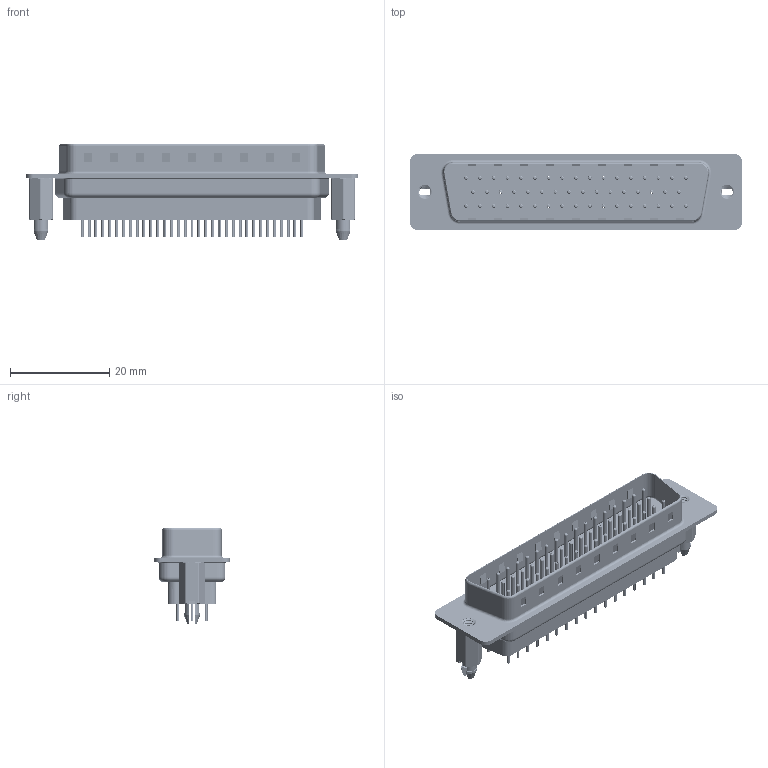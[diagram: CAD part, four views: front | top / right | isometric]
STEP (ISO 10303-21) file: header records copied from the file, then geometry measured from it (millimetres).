
FILE_DESCRIPTION (( 'STEP AP203' ), '1' );
FILE_NAME ('627-050-228-266.STEP', '2020-07-21T18:28:10', ( '' ), ( '' ), 'SwSTEP 2.0', 'SolidWorks 2020', '' );
FILE_SCHEMA (( 'CONFIG_CONTROL_DESIGN' ));
Length unit declared in the file: millimetre
Products named in the file (8): 627 Shell Front_50 Contacts; 627 Housing_50 FF; 627 Contact Row 2_28L; 627 Shell Rear_50 Contacts; 627 Contact Row 3_28L; 627 Contact Row 1_28L; 627 4-40 Threaded Boardlock_FF; 627-050-228-266
Assembly tree (55 placements, depth 2):
  627-050-228-266
    627 Housing_50 FF
    627 Shell Front_50 Contacts
    627 Shell Rear_50 Contacts
    627 Contact Row 1_28L  x17
    627 Contact Row 2_28L  x16
    627 Contact Row 3_28L  x17
    627 4-40 Threaded Boardlock_FF  x2
Bounding box: 67 x 15.3 x 19.4 mm (x, y, z)
Volume: 5736 mm3; surface area: 15095.9 mm2
Topology: 56 solids, 56 shells, 5579 faces, 14710 edges, 9152 vertices
Faces by surface type: cylinder 2162, plane 1441, torus 1406, cone 516, bspline 54
Entity records: 56639 total; most frequent: CARTESIAN_POINT 23218, DIRECTION 6902, ORIENTED_EDGE 6292, EDGE_CURVE 3146, AXIS2_PLACEMENT_3D 2763, VERTEX_POINT 2032, EDGE_LOOP 1596, CIRCLE 1494
